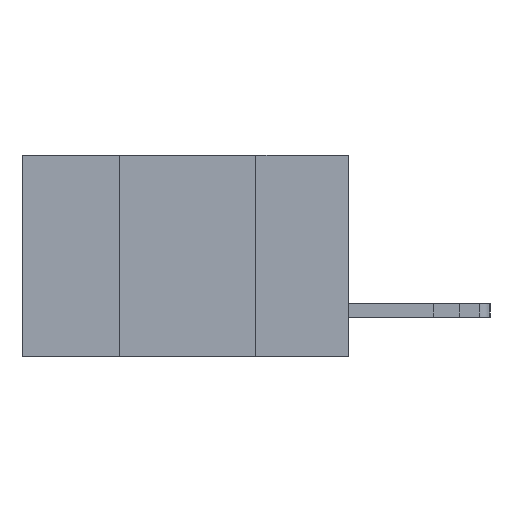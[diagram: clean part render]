
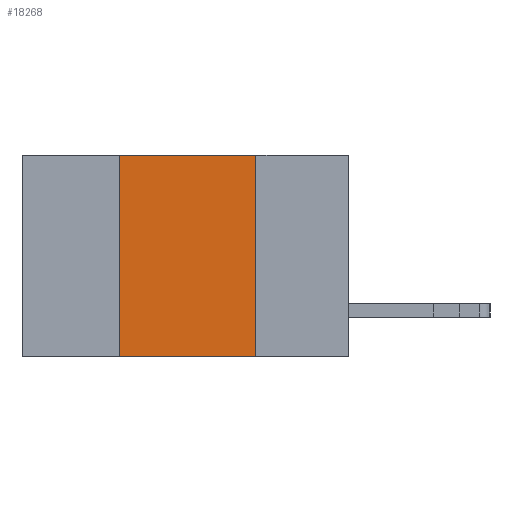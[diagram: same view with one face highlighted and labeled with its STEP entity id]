
A CAD part, left-side view. The second image highlights one B-rep face of the part: STEP entity #18268.
In plain terms, the highlighted planar face has unit normal (-1, 0, 0).
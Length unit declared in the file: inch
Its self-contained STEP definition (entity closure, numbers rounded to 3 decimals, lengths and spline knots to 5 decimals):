
#209 = EDGE_LOOP ( 'NONE', ( #1948, #10180, #12255, #16616 ) ) ;
#777 = DIRECTION ( 'NONE',  ( 0., -1., 0. ) ) ;
#966 = CARTESIAN_POINT ( 'NONE',  ( 0., 0.6, 0. ) ) ;
#1858 = DIRECTION ( 'NONE',  ( 0., 0., -1. ) ) ;
#1948 = ORIENTED_EDGE ( 'NONE', *, *, #17114, .F. ) ;
#4070 = DIRECTION ( 'NONE',  ( 0., 0., 1. ) ) ;
#4444 = CARTESIAN_POINT ( 'NONE',  ( 0., 0.42, 0. ) ) ;
#4641 = VECTOR ( 'NONE', #777, 39.37008 ) ;
#4937 = VERTEX_POINT ( 'NONE', #13172 ) ;
#5454 = CARTESIAN_POINT ( 'NONE',  ( 0., 0.42, -0.37 ) ) ;
#6413 = VECTOR ( 'NONE', #8422, 39.37008 ) ;
#6748 = CARTESIAN_POINT ( 'NONE',  ( 0., 0.17, -0.37 ) ) ;
#6835 = CARTESIAN_POINT ( 'NONE',  ( 0., 0.17, 0. ) ) ;
#8011 = VERTEX_POINT ( 'NONE', #6748 ) ;
#8268 = CARTESIAN_POINT ( 'NONE',  ( 0., 0.6, 0. ) ) ;
#8272 = EDGE_CURVE ( 'NONE', #15598, #4937, #12896, .T. ) ;
#8422 = DIRECTION ( 'NONE',  ( 0., 0., -1. ) ) ;
#8741 = DIRECTION ( 'NONE',  ( 0., -1., 0. ) ) ;
#8807 = CARTESIAN_POINT ( 'NONE',  ( 0., 0.6, -0.37 ) ) ;
#9353 = LINE ( 'NONE', #13420, #13951 ) ;
#9482 = EDGE_CURVE ( 'NONE', #17778, #8011, #17433, .T. ) ;
#10180 = ORIENTED_EDGE ( 'NONE', *, *, #8272, .F. ) ;
#10751 = AXIS2_PLACEMENT_3D ( 'NONE', #8268, #11350, #1858 ) ;
#11350 = DIRECTION ( 'NONE',  ( 1., 0., 0. ) ) ;
#12255 = ORIENTED_EDGE ( 'NONE', *, *, #16089, .F. ) ;
#12896 = LINE ( 'NONE', #966, #4641 ) ;
#13172 = CARTESIAN_POINT ( 'NONE',  ( 0., 0.17, 0. ) ) ;
#13349 = VECTOR ( 'NONE', #8741, 39.37008 ) ;
#13420 = CARTESIAN_POINT ( 'NONE',  ( 0., 0.42, 0. ) ) ;
#13951 = VECTOR ( 'NONE', #4070, 39.37008 ) ;
#15598 = VERTEX_POINT ( 'NONE', #4444 ) ;
#16036 = FACE_OUTER_BOUND ( 'NONE', #209, .T. ) ;
#16089 = EDGE_CURVE ( 'NONE', #17778, #15598, #9353, .T. ) ;
#16616 = ORIENTED_EDGE ( 'NONE', *, *, #9482, .T. ) ;
#17114 = EDGE_CURVE ( 'NONE', #4937, #8011, #18202, .T. ) ;
#17433 = LINE ( 'NONE', #8807, #13349 ) ;
#17467 = PLANE ( 'NONE',  #10751 ) ;
#17778 = VERTEX_POINT ( 'NONE', #5454 ) ;
#18202 = LINE ( 'NONE', #6835, #6413 ) ;
#18268 = ADVANCED_FACE ( 'NONE', ( #16036 ), #17467, .F. ) ;
